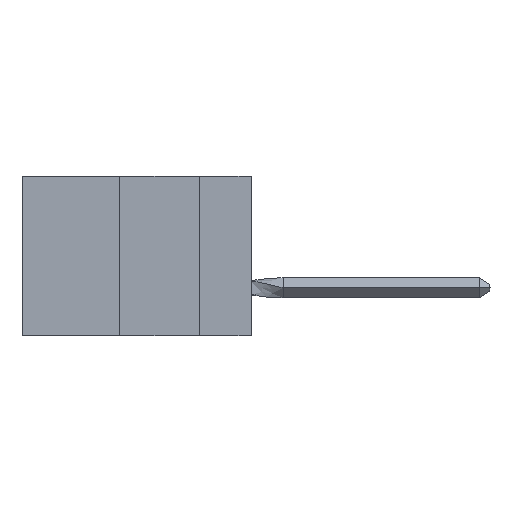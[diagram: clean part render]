
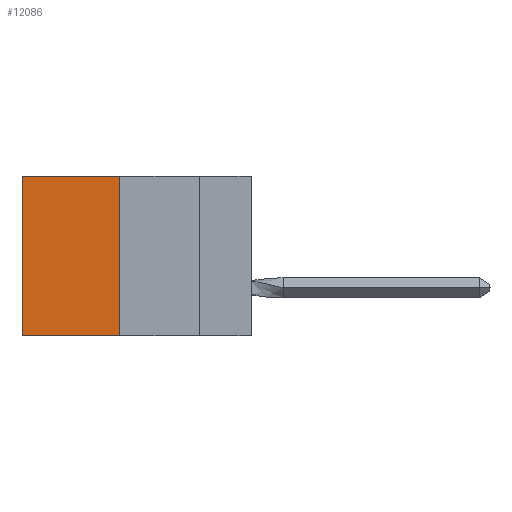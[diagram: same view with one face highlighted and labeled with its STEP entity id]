
A CAD part, left-side view. The second image highlights one B-rep face of the part: STEP entity #12086.
In plain terms, the highlighted planar face has unit normal (-1, 0, 0).
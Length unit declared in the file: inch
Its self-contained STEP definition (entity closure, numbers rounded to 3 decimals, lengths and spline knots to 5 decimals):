
#863 = DIRECTION ( 'NONE',  ( 0., 1., 0. ) ) ;
#1309 = VECTOR ( 'NONE', #22375, 39.37008 ) ;
#1928 = CARTESIAN_POINT ( 'NONE',  ( 0.305, 0.413, 0. ) ) ;
#4966 = VECTOR ( 'NONE', #8030, 39.37008 ) ;
#5256 = ORIENTED_EDGE ( 'NONE', *, *, #12191, .T. ) ;
#5269 = AXIS2_PLACEMENT_3D ( 'NONE', #17719, #26172, #8994 ) ;
#6211 = ORIENTED_EDGE ( 'NONE', *, *, #22054, .F. ) ;
#6473 = FACE_OUTER_BOUND ( 'NONE', #11923, .T. ) ;
#6675 = VERTEX_POINT ( 'NONE', #12394 ) ;
#6875 = CARTESIAN_POINT ( 'NONE',  ( 0.305, 0.72, -0.5 ) ) ;
#8030 = DIRECTION ( 'NONE',  ( 0., 0., -1. ) ) ;
#8994 = DIRECTION ( 'NONE',  ( 0., 0., -1. ) ) ;
#9088 = PLANE ( 'NONE',  #5269 ) ;
#11399 = VERTEX_POINT ( 'NONE', #1928 ) ;
#11923 = EDGE_LOOP ( 'NONE', ( #22124, #21986, #6211, #5256 ) ) ;
#12086 = ADVANCED_FACE ( 'NONE', ( #6473 ), #9088, .F. ) ;
#12191 = EDGE_CURVE ( 'NONE', #11399, #6675, #19680, .T. ) ;
#12394 = CARTESIAN_POINT ( 'NONE',  ( 0.305, 0.72, 0. ) ) ;
#12750 = VERTEX_POINT ( 'NONE', #24513 ) ;
#14021 = DIRECTION ( 'NONE',  ( 0., 1., 0. ) ) ;
#14293 = EDGE_CURVE ( 'NONE', #25338, #12750, #23592, .T. ) ;
#17719 = CARTESIAN_POINT ( 'NONE',  ( 0.305, 0.413, -0.5 ) ) ;
#17894 = VECTOR ( 'NONE', #863, 39.37008 ) ;
#18210 = CARTESIAN_POINT ( 'NONE',  ( 0.305, 0.413, -0.5 ) ) ;
#19680 = LINE ( 'NONE', #27065, #26103 ) ;
#21684 = EDGE_CURVE ( 'NONE', #6675, #12750, #22073, .T. ) ;
#21986 = ORIENTED_EDGE ( 'NONE', *, *, #14293, .F. ) ;
#22054 = EDGE_CURVE ( 'NONE', #11399, #25338, #23405, .T. ) ;
#22073 = LINE ( 'NONE', #6875, #1309 ) ;
#22124 = ORIENTED_EDGE ( 'NONE', *, *, #21684, .T. ) ;
#22375 = DIRECTION ( 'NONE',  ( 0., 0., -1. ) ) ;
#23405 = LINE ( 'NONE', #24926, #4966 ) ;
#23592 = LINE ( 'NONE', #26273, #17894 ) ;
#24513 = CARTESIAN_POINT ( 'NONE',  ( 0.305, 0.72, -0.5 ) ) ;
#24926 = CARTESIAN_POINT ( 'NONE',  ( 0.305, 0.413, -0.5 ) ) ;
#25338 = VERTEX_POINT ( 'NONE', #18210 ) ;
#26103 = VECTOR ( 'NONE', #14021, 39.37008 ) ;
#26172 = DIRECTION ( 'NONE',  ( 1., 0., 0. ) ) ;
#26273 = CARTESIAN_POINT ( 'NONE',  ( 0.305, 0.413, -0.5 ) ) ;
#27065 = CARTESIAN_POINT ( 'NONE',  ( 0.305, 0.413, 0. ) ) ;
